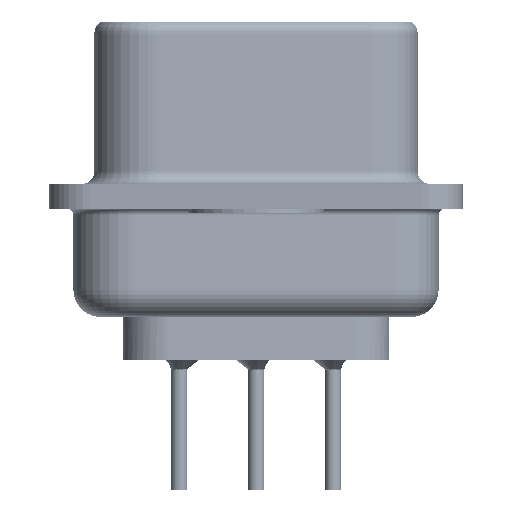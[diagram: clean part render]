
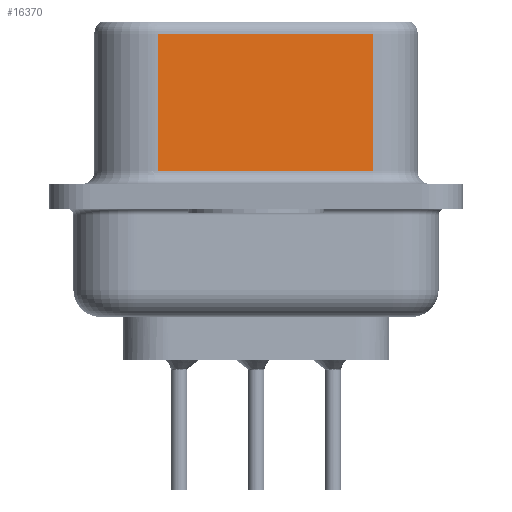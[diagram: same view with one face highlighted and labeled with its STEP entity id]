
A CAD part, left-side view. The second image highlights one B-rep face of the part: STEP entity #16370.
In plain terms, the highlighted planar face has unit normal (-0.985, -0.174, 0).
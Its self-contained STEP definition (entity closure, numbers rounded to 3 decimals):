
#154 = DIRECTION ( 'NONE',  ( 0.174, -0.985, 0. ) ) ;
#449 = PLANE ( 'NONE',  #17832 ) ;
#1156 = DIRECTION ( 'NONE',  ( -0.174, 0.985, 0. ) ) ;
#1858 = VECTOR ( 'NONE', #24692, 1000. ) ;
#2859 = VERTEX_POINT ( 'NONE', #23813 ) ;
#3060 = CARTESIAN_POINT ( 'NONE',  ( 5.132, -4.322, 6.52 ) ) ;
#3144 = CARTESIAN_POINT ( 'NONE',  ( 5.132, -4.322, 6.52 ) ) ;
#3231 = FACE_OUTER_BOUND ( 'NONE', #20457, .T. ) ;
#4753 = EDGE_CURVE ( 'NONE', #2859, #13731, #29692, .T. ) ;
#6193 = CARTESIAN_POINT ( 'NONE',  ( 3.73, 3.628, 6.52 ) ) ;
#6314 = CARTESIAN_POINT ( 'NONE',  ( 5.132, -4.322, 0.95 ) ) ;
#7113 = ORIENTED_EDGE ( 'NONE', *, *, #7497, .T. ) ;
#7497 = EDGE_CURVE ( 'NONE', #16304, #14546, #20902, .T. ) ;
#11022 = LINE ( 'NONE', #6193, #1858 ) ;
#13115 = CARTESIAN_POINT ( 'NONE',  ( 5.132, -4.322, 0.95 ) ) ;
#13332 = DIRECTION ( 'NONE',  ( 0., 0., -1. ) ) ;
#13731 = VERTEX_POINT ( 'NONE', #25080 ) ;
#14546 = VERTEX_POINT ( 'NONE', #6314 ) ;
#16304 = VERTEX_POINT ( 'NONE', #31944 ) ;
#16370 = ADVANCED_FACE ( 'NONE', ( #3231 ), #449, .F. ) ;
#16690 = DIRECTION ( 'NONE',  ( 0.985, 0.174, 0. ) ) ;
#16858 = VECTOR ( 'NONE', #13332, 1000. ) ;
#17832 = AXIS2_PLACEMENT_3D ( 'NONE', #3060, #16690, #30025 ) ;
#19471 = CARTESIAN_POINT ( 'NONE',  ( 5.132, -4.322, 6.02 ) ) ;
#19983 = ORIENTED_EDGE ( 'NONE', *, *, #31057, .T. ) ;
#20457 = EDGE_LOOP ( 'NONE', ( #29792, #20499, #19983, #7113 ) ) ;
#20499 = ORIENTED_EDGE ( 'NONE', *, *, #4753, .T. ) ;
#20902 = LINE ( 'NONE', #13115, #23991 ) ;
#23813 = CARTESIAN_POINT ( 'NONE',  ( 5.132, -4.322, 6.02 ) ) ;
#23991 = VECTOR ( 'NONE', #154, 1000. ) ;
#24692 = DIRECTION ( 'NONE',  ( 0., 0., -1. ) ) ;
#25080 = CARTESIAN_POINT ( 'NONE',  ( 3.73, 3.628, 6.02 ) ) ;
#28441 = VECTOR ( 'NONE', #1156, 1000. ) ;
#29094 = LINE ( 'NONE', #3144, #16858 ) ;
#29692 = LINE ( 'NONE', #19471, #28441 ) ;
#29792 = ORIENTED_EDGE ( 'NONE', *, *, #32993, .F. ) ;
#30025 = DIRECTION ( 'NONE',  ( -0.174, 0.985, 0. ) ) ;
#31057 = EDGE_CURVE ( 'NONE', #13731, #16304, #11022, .T. ) ;
#31944 = CARTESIAN_POINT ( 'NONE',  ( 3.73, 3.628, 0.95 ) ) ;
#32993 = EDGE_CURVE ( 'NONE', #2859, #14546, #29094, .T. ) ;
